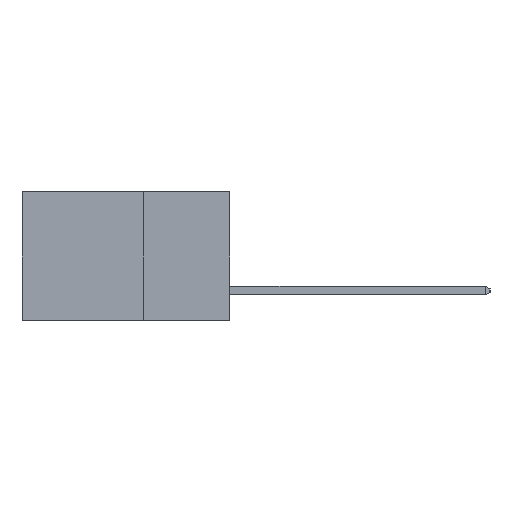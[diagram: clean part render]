
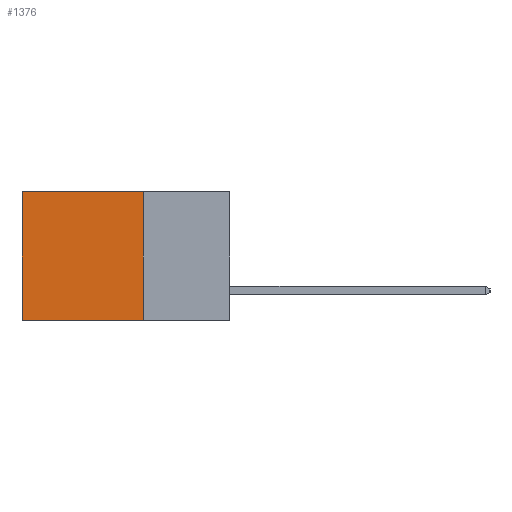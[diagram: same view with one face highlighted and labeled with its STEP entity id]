
A CAD part, left-side view. The second image highlights one B-rep face of the part: STEP entity #1376.
In plain terms, the highlighted planar face has unit normal (-1, 0, 0).
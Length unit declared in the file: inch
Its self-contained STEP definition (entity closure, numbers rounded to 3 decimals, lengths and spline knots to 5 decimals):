
#257 = FACE_OUTER_BOUND ( 'NONE', #6624, .T. ) ;
#1376 = ADVANCED_FACE ( 'NONE', ( #257 ), #19948, .F. ) ;
#1944 = CARTESIAN_POINT ( 'NONE',  ( 0.2615, 0.25, -0.37 ) ) ;
#2009 = CARTESIAN_POINT ( 'NONE',  ( 0.2615, 0.25, 0. ) ) ;
#2031 = VECTOR ( 'NONE', #23402, 39.37008 ) ;
#2372 = ORIENTED_EDGE ( 'NONE', *, *, #16905, .F. ) ;
#3299 = ORIENTED_EDGE ( 'NONE', *, *, #24622, .T. ) ;
#3815 = VECTOR ( 'NONE', #13196, 39.37008 ) ;
#4683 = VECTOR ( 'NONE', #18129, 39.37008 ) ;
#4882 = EDGE_CURVE ( 'NONE', #16234, #17487, #8483, .T. ) ;
#5137 = CARTESIAN_POINT ( 'NONE',  ( 0.2615, 0.25, -0.37 ) ) ;
#6624 = EDGE_LOOP ( 'NONE', ( #23841, #2372, #16376, #3299 ) ) ;
#8483 = LINE ( 'NONE', #13440, #3815 ) ;
#9397 = LINE ( 'NONE', #21987, #4683 ) ;
#13196 = DIRECTION ( 'NONE',  ( 0., 0., -1. ) ) ;
#13440 = CARTESIAN_POINT ( 'NONE',  ( 0.2615, 0.6, -0.37 ) ) ;
#13774 = DIRECTION ( 'NONE',  ( 0., 0., -1. ) ) ;
#15076 = VERTEX_POINT ( 'NONE', #18212 ) ;
#16164 = EDGE_CURVE ( 'NONE', #15076, #19789, #17306, .T. ) ;
#16234 = VERTEX_POINT ( 'NONE', #17738 ) ;
#16376 = ORIENTED_EDGE ( 'NONE', *, *, #16164, .F. ) ;
#16905 = EDGE_CURVE ( 'NONE', #19789, #17487, #9397, .T. ) ;
#17274 = AXIS2_PLACEMENT_3D ( 'NONE', #19387, #18943, #18277 ) ;
#17306 = LINE ( 'NONE', #1944, #21233 ) ;
#17487 = VERTEX_POINT ( 'NONE', #17854 ) ;
#17706 = LINE ( 'NONE', #2009, #2031 ) ;
#17738 = CARTESIAN_POINT ( 'NONE',  ( 0.2615, 0.6, 0. ) ) ;
#17854 = CARTESIAN_POINT ( 'NONE',  ( 0.2615, 0.6, -0.37 ) ) ;
#18129 = DIRECTION ( 'NONE',  ( 0., 1., 0. ) ) ;
#18212 = CARTESIAN_POINT ( 'NONE',  ( 0.2615, 0.25, 0. ) ) ;
#18277 = DIRECTION ( 'NONE',  ( 0., 0., -1. ) ) ;
#18943 = DIRECTION ( 'NONE',  ( 1., 0., 0. ) ) ;
#19387 = CARTESIAN_POINT ( 'NONE',  ( 0.2615, 0.25, -0.37 ) ) ;
#19789 = VERTEX_POINT ( 'NONE', #5137 ) ;
#19948 = PLANE ( 'NONE',  #17274 ) ;
#21233 = VECTOR ( 'NONE', #13774, 39.37008 ) ;
#21987 = CARTESIAN_POINT ( 'NONE',  ( 0.2615, 0.25, -0.37 ) ) ;
#23402 = DIRECTION ( 'NONE',  ( 0., 1., 0. ) ) ;
#23841 = ORIENTED_EDGE ( 'NONE', *, *, #4882, .T. ) ;
#24622 = EDGE_CURVE ( 'NONE', #15076, #16234, #17706, .T. ) ;
